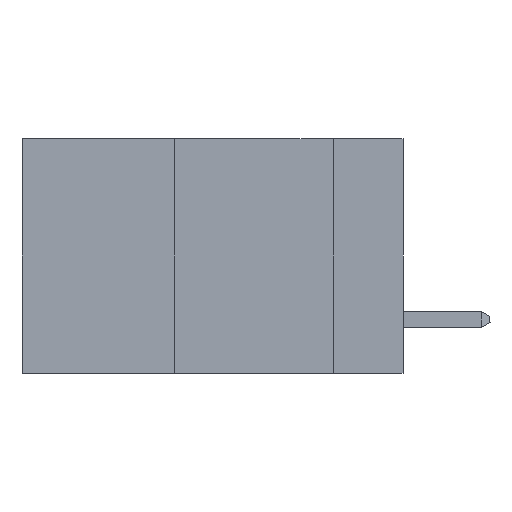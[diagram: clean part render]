
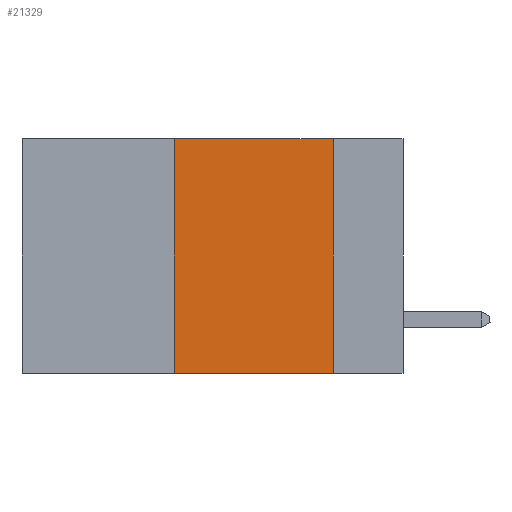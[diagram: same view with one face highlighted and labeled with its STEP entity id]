
A CAD part, left-side view. The second image highlights one B-rep face of the part: STEP entity #21329.
In plain terms, the highlighted planar face has unit normal (-1, 0, 0).
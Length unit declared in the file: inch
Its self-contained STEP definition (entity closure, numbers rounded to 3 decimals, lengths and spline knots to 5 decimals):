
#5 = ORIENTED_EDGE ( 'NONE', *, *, #8132, .F. ) ;
#470 = LINE ( 'NONE', #8075, #17643 ) ;
#1057 = DIRECTION ( 'NONE',  ( 0., 0., -1. ) ) ;
#1115 = EDGE_CURVE ( 'NONE', #17487, #15663, #9972, .T. ) ;
#1532 = CARTESIAN_POINT ( 'NONE',  ( 0., 0.6, -0.37 ) ) ;
#2505 = ORIENTED_EDGE ( 'NONE', *, *, #1115, .T. ) ;
#2786 = CARTESIAN_POINT ( 'NONE',  ( 0., 0.11, -0.37 ) ) ;
#3040 = CARTESIAN_POINT ( 'NONE',  ( 0., 0.36, 0. ) ) ;
#3382 = CARTESIAN_POINT ( 'NONE',  ( 0., 0.11, 0. ) ) ;
#6757 = VERTEX_POINT ( 'NONE', #3382 ) ;
#6797 = LINE ( 'NONE', #17453, #15842 ) ;
#8075 = CARTESIAN_POINT ( 'NONE',  ( 0., 0.36, 0. ) ) ;
#8132 = EDGE_CURVE ( 'NONE', #17487, #14545, #470, .T. ) ;
#8725 = DIRECTION ( 'NONE',  ( 0., 0., -1. ) ) ;
#9399 = VECTOR ( 'NONE', #10429, 39.37008 ) ;
#9916 = EDGE_CURVE ( 'NONE', #6757, #15663, #6797, .T. ) ;
#9972 = LINE ( 'NONE', #1532, #9399 ) ;
#10290 = VECTOR ( 'NONE', #18596, 39.37008 ) ;
#10429 = DIRECTION ( 'NONE',  ( 0., -1., 0. ) ) ;
#11251 = ORIENTED_EDGE ( 'NONE', *, *, #12095, .F. ) ;
#11584 = EDGE_LOOP ( 'NONE', ( #13542, #11251, #5, #2505 ) ) ;
#12095 = EDGE_CURVE ( 'NONE', #14545, #6757, #14914, .T. ) ;
#12239 = PLANE ( 'NONE',  #20669 ) ;
#13050 = CARTESIAN_POINT ( 'NONE',  ( 0., 0.6, 0. ) ) ;
#13381 = CARTESIAN_POINT ( 'NONE',  ( 0., 0.36, -0.37 ) ) ;
#13542 = ORIENTED_EDGE ( 'NONE', *, *, #9916, .F. ) ;
#14068 = DIRECTION ( 'NONE',  ( 1., 0., 0. ) ) ;
#14545 = VERTEX_POINT ( 'NONE', #3040 ) ;
#14914 = LINE ( 'NONE', #13050, #10290 ) ;
#15663 = VERTEX_POINT ( 'NONE', #2786 ) ;
#15842 = VECTOR ( 'NONE', #1057, 39.37008 ) ;
#17453 = CARTESIAN_POINT ( 'NONE',  ( 0., 0.11, 0. ) ) ;
#17487 = VERTEX_POINT ( 'NONE', #13381 ) ;
#17643 = VECTOR ( 'NONE', #21965, 39.37008 ) ;
#18596 = DIRECTION ( 'NONE',  ( 0., -1., 0. ) ) ;
#20669 = AXIS2_PLACEMENT_3D ( 'NONE', #21041, #14068, #8725 ) ;
#21041 = CARTESIAN_POINT ( 'NONE',  ( 0., 0.6, 0. ) ) ;
#21329 = ADVANCED_FACE ( 'NONE', ( #21434 ), #12239, .F. ) ;
#21434 = FACE_OUTER_BOUND ( 'NONE', #11584, .T. ) ;
#21965 = DIRECTION ( 'NONE',  ( 0., 0., 1. ) ) ;
